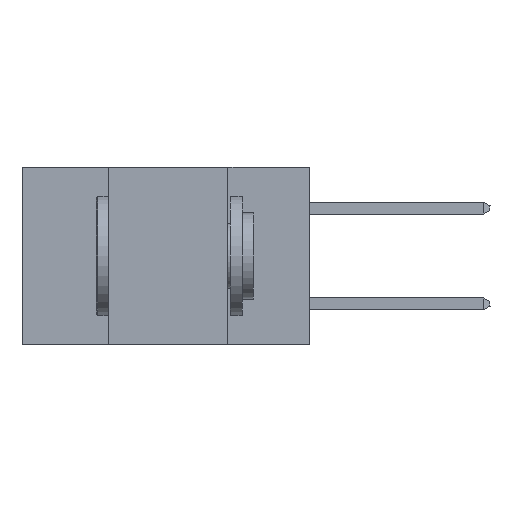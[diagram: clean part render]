
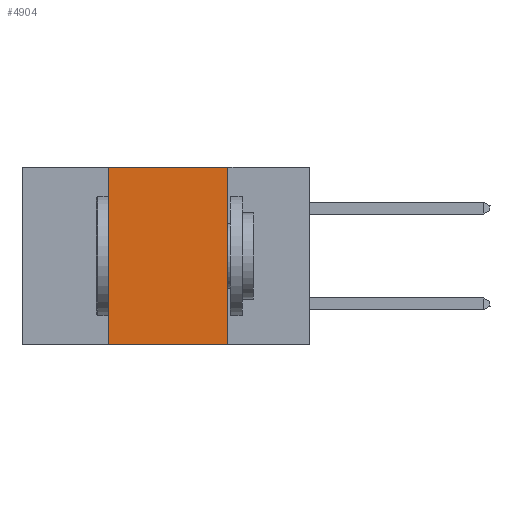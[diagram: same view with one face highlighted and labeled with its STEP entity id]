
A CAD part, left-side view. The second image highlights one B-rep face of the part: STEP entity #4904.
In plain terms, the highlighted planar face has unit normal (-1, 0, 0).
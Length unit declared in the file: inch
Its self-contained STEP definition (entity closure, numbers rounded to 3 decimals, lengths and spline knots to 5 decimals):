
#26 = DIRECTION ( 'NONE',  ( 0., 0., 1. ) ) ;
#437 = CARTESIAN_POINT ( 'NONE',  ( 0., 0.42, 0. ) ) ;
#592 = VECTOR ( 'NONE', #4704, 39.37008 ) ;
#985 = LINE ( 'NONE', #5396, #19097 ) ;
#1419 = VERTEX_POINT ( 'NONE', #437 ) ;
#1564 = VERTEX_POINT ( 'NONE', #8449 ) ;
#1610 = VERTEX_POINT ( 'NONE', #8521 ) ;
#2222 = LINE ( 'NONE', #16975, #592 ) ;
#4195 = ORIENTED_EDGE ( 'NONE', *, *, #17375, .F. ) ;
#4643 = CARTESIAN_POINT ( 'NONE',  ( 0., 0.6, 0. ) ) ;
#4704 = DIRECTION ( 'NONE',  ( 0., -1., 0. ) ) ;
#4904 = ADVANCED_FACE ( 'NONE', ( #17413 ), #10255, .F. ) ;
#4951 = VECTOR ( 'NONE', #22084, 39.37008 ) ;
#5396 = CARTESIAN_POINT ( 'NONE',  ( 0., 0.17, 0. ) ) ;
#6173 = EDGE_CURVE ( 'NONE', #7385, #1419, #7191, .T. ) ;
#6718 = CARTESIAN_POINT ( 'NONE',  ( 0., 0.42, -0.37 ) ) ;
#7191 = LINE ( 'NONE', #8757, #11318 ) ;
#7213 = EDGE_CURVE ( 'NONE', #1419, #1564, #9610, .T. ) ;
#7385 = VERTEX_POINT ( 'NONE', #6718 ) ;
#8449 = CARTESIAN_POINT ( 'NONE',  ( 0., 0.17, 0. ) ) ;
#8521 = CARTESIAN_POINT ( 'NONE',  ( 0., 0.17, -0.37 ) ) ;
#8667 = ORIENTED_EDGE ( 'NONE', *, *, #22690, .T. ) ;
#8757 = CARTESIAN_POINT ( 'NONE',  ( 0., 0.42, 0. ) ) ;
#9610 = LINE ( 'NONE', #4643, #4951 ) ;
#10255 = PLANE ( 'NONE',  #15584 ) ;
#11318 = VECTOR ( 'NONE', #26, 39.37008 ) ;
#12379 = DIRECTION ( 'NONE',  ( 1., 0., 0. ) ) ;
#12530 = EDGE_LOOP ( 'NONE', ( #4195, #15473, #14428, #8667 ) ) ;
#14232 = DIRECTION ( 'NONE',  ( 0., 0., -1. ) ) ;
#14428 = ORIENTED_EDGE ( 'NONE', *, *, #6173, .F. ) ;
#15473 = ORIENTED_EDGE ( 'NONE', *, *, #7213, .F. ) ;
#15584 = AXIS2_PLACEMENT_3D ( 'NONE', #19425, #12379, #14232 ) ;
#16975 = CARTESIAN_POINT ( 'NONE',  ( 0., 0.6, -0.37 ) ) ;
#17375 = EDGE_CURVE ( 'NONE', #1564, #1610, #985, .T. ) ;
#17413 = FACE_OUTER_BOUND ( 'NONE', #12530, .T. ) ;
#19097 = VECTOR ( 'NONE', #21514, 39.37008 ) ;
#19425 = CARTESIAN_POINT ( 'NONE',  ( 0., 0.6, 0. ) ) ;
#21514 = DIRECTION ( 'NONE',  ( 0., 0., -1. ) ) ;
#22084 = DIRECTION ( 'NONE',  ( 0., -1., 0. ) ) ;
#22690 = EDGE_CURVE ( 'NONE', #7385, #1610, #2222, .T. ) ;
